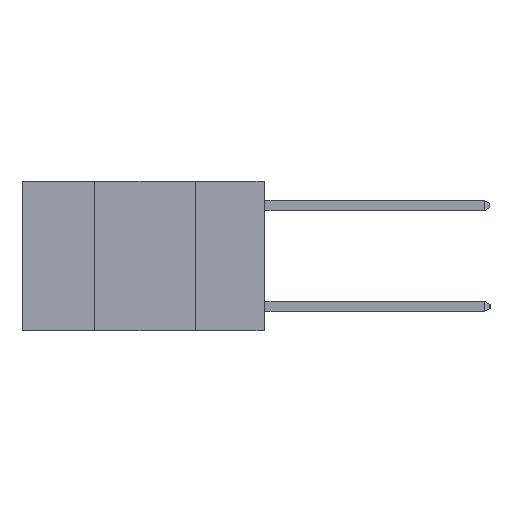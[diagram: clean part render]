
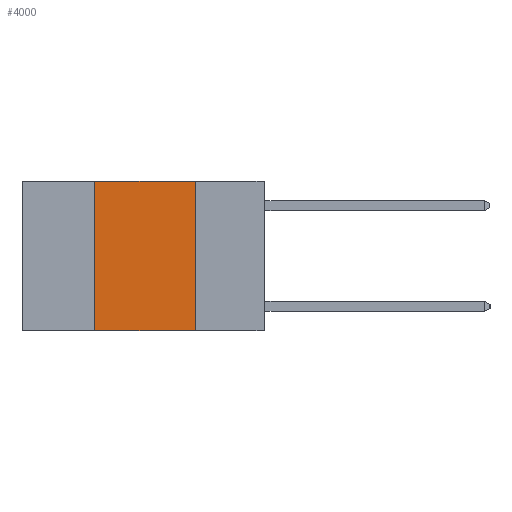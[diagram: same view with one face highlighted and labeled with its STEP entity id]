
A CAD part, left-side view. The second image highlights one B-rep face of the part: STEP entity #4000.
In plain terms, the highlighted planar face has unit normal (-1, 0, 0).
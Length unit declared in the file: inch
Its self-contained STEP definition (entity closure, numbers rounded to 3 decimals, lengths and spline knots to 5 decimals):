
#23 = CARTESIAN_POINT ( 'NONE',  ( 0., 0.42, 0. ) ) ;
#188 = VECTOR ( 'NONE', #2131, 39.37008 ) ;
#844 = VERTEX_POINT ( 'NONE', #7332 ) ;
#1032 = VERTEX_POINT ( 'NONE', #23 ) ;
#1143 = LINE ( 'NONE', #7280, #4695 ) ;
#1278 = LINE ( 'NONE', #1526, #2916 ) ;
#1526 = CARTESIAN_POINT ( 'NONE',  ( 0., 0.6, -0.37 ) ) ;
#1617 = CARTESIAN_POINT ( 'NONE',  ( 0., 0.17, 0. ) ) ;
#1934 = EDGE_LOOP ( 'NONE', ( #4363, #5441, #4969, #6410 ) ) ;
#2131 = DIRECTION ( 'NONE',  ( 0., 0., -1. ) ) ;
#2416 = CARTESIAN_POINT ( 'NONE',  ( 0., 0.6, 0. ) ) ;
#2611 = AXIS2_PLACEMENT_3D ( 'NONE', #5698, #5495, #5489 ) ;
#2916 = VECTOR ( 'NONE', #6876, 39.37008 ) ;
#3139 = DIRECTION ( 'NONE',  ( 0., -1., 0. ) ) ;
#3187 = EDGE_CURVE ( 'NONE', #844, #5079, #1278, .T. ) ;
#3216 = VERTEX_POINT ( 'NONE', #1617 ) ;
#3567 = LINE ( 'NONE', #2416, #7041 ) ;
#3654 = EDGE_CURVE ( 'NONE', #844, #1032, #1143, .T. ) ;
#4000 = ADVANCED_FACE ( 'NONE', ( #4251 ), #5581, .F. ) ;
#4251 = FACE_OUTER_BOUND ( 'NONE', #1934, .T. ) ;
#4363 = ORIENTED_EDGE ( 'NONE', *, *, #4619, .F. ) ;
#4619 = EDGE_CURVE ( 'NONE', #3216, #5079, #5620, .T. ) ;
#4695 = VECTOR ( 'NONE', #7264, 39.37008 ) ;
#4969 = ORIENTED_EDGE ( 'NONE', *, *, #3654, .F. ) ;
#5079 = VERTEX_POINT ( 'NONE', #8708 ) ;
#5384 = EDGE_CURVE ( 'NONE', #1032, #3216, #3567, .T. ) ;
#5441 = ORIENTED_EDGE ( 'NONE', *, *, #5384, .F. ) ;
#5489 = DIRECTION ( 'NONE',  ( 0., 0., -1. ) ) ;
#5495 = DIRECTION ( 'NONE',  ( 1., 0., 0. ) ) ;
#5581 = PLANE ( 'NONE',  #2611 ) ;
#5620 = LINE ( 'NONE', #5663, #188 ) ;
#5663 = CARTESIAN_POINT ( 'NONE',  ( 0., 0.17, 0. ) ) ;
#5698 = CARTESIAN_POINT ( 'NONE',  ( 0., 0.6, 0. ) ) ;
#6410 = ORIENTED_EDGE ( 'NONE', *, *, #3187, .T. ) ;
#6876 = DIRECTION ( 'NONE',  ( 0., -1., 0. ) ) ;
#7041 = VECTOR ( 'NONE', #3139, 39.37008 ) ;
#7264 = DIRECTION ( 'NONE',  ( 0., 0., 1. ) ) ;
#7280 = CARTESIAN_POINT ( 'NONE',  ( 0., 0.42, 0. ) ) ;
#7332 = CARTESIAN_POINT ( 'NONE',  ( 0., 0.42, -0.37 ) ) ;
#8708 = CARTESIAN_POINT ( 'NONE',  ( 0., 0.17, -0.37 ) ) ;
